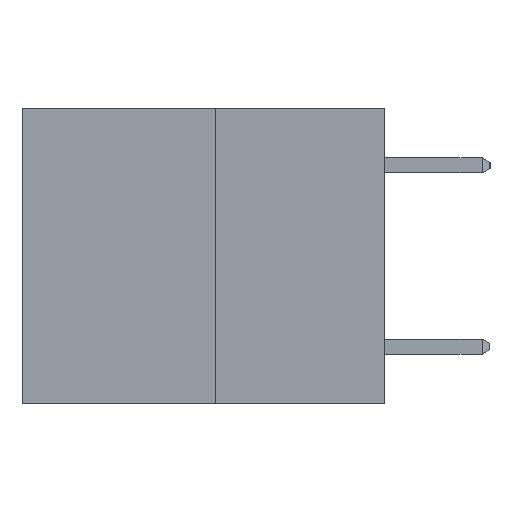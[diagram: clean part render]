
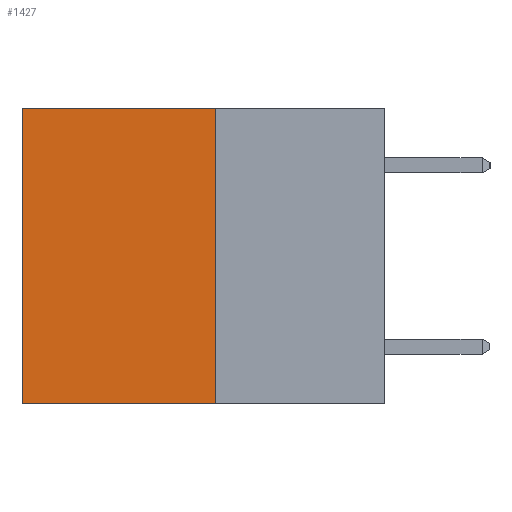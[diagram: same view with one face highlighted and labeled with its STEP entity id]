
A CAD part, left-side view. The second image highlights one B-rep face of the part: STEP entity #1427.
In plain terms, the highlighted planar face has unit normal (-1, 0, 0).
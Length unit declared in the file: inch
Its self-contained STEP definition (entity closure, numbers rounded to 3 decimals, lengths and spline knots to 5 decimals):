
#257 = CARTESIAN_POINT ( 'NONE',  ( 0.3165, 0.6, -0.49 ) ) ;
#453 = CARTESIAN_POINT ( 'NONE',  ( 0.3165, 0.28, 0. ) ) ;
#1127 = PLANE ( 'NONE',  #2078 ) ;
#1200 = LINE ( 'NONE', #2493, #6052 ) ;
#1427 = ADVANCED_FACE ( 'NONE', ( #3220 ), #1127, .F. ) ;
#1482 = EDGE_CURVE ( 'NONE', #6017, #5629, #5645, .T. ) ;
#1552 = ORIENTED_EDGE ( 'NONE', *, *, #5616, .T. ) ;
#2078 = AXIS2_PLACEMENT_3D ( 'NONE', #8502, #3568, #4407 ) ;
#2493 = CARTESIAN_POINT ( 'NONE',  ( 0.3165, 0.28, -0.49 ) ) ;
#3220 = FACE_OUTER_BOUND ( 'NONE', #8354, .T. ) ;
#3568 = DIRECTION ( 'NONE',  ( 1., 0., 0. ) ) ;
#4062 = DIRECTION ( 'NONE',  ( 0., 0., -1. ) ) ;
#4073 = CARTESIAN_POINT ( 'NONE',  ( 0.3165, 0.28, -0.49 ) ) ;
#4407 = DIRECTION ( 'NONE',  ( 0., 0., -1. ) ) ;
#4700 = CARTESIAN_POINT ( 'NONE',  ( 0.3165, 0.6, -0.49 ) ) ;
#4723 = VERTEX_POINT ( 'NONE', #453 ) ;
#4753 = LINE ( 'NONE', #8108, #9536 ) ;
#5454 = LINE ( 'NONE', #4073, #7257 ) ;
#5616 = EDGE_CURVE ( 'NONE', #4723, #6017, #4753, .T. ) ;
#5629 = VERTEX_POINT ( 'NONE', #257 ) ;
#5645 = LINE ( 'NONE', #4700, #7568 ) ;
#5780 = EDGE_CURVE ( 'NONE', #4723, #6565, #1200, .T. ) ;
#6017 = VERTEX_POINT ( 'NONE', #7781 ) ;
#6052 = VECTOR ( 'NONE', #4062, 39.37008 ) ;
#6565 = VERTEX_POINT ( 'NONE', #8383 ) ;
#6800 = EDGE_CURVE ( 'NONE', #6565, #5629, #5454, .T. ) ;
#7257 = VECTOR ( 'NONE', #8183, 39.37008 ) ;
#7568 = VECTOR ( 'NONE', #10477, 39.37008 ) ;
#7781 = CARTESIAN_POINT ( 'NONE',  ( 0.3165, 0.6, 0. ) ) ;
#8108 = CARTESIAN_POINT ( 'NONE',  ( 0.3165, 0.28, 0. ) ) ;
#8158 = DIRECTION ( 'NONE',  ( 0., 1., 0. ) ) ;
#8183 = DIRECTION ( 'NONE',  ( 0., 1., 0. ) ) ;
#8354 = EDGE_LOOP ( 'NONE', ( #9831, #10308, #9812, #1552 ) ) ;
#8383 = CARTESIAN_POINT ( 'NONE',  ( 0.3165, 0.28, -0.49 ) ) ;
#8502 = CARTESIAN_POINT ( 'NONE',  ( 0.3165, 0.28, -0.49 ) ) ;
#9536 = VECTOR ( 'NONE', #8158, 39.37008 ) ;
#9812 = ORIENTED_EDGE ( 'NONE', *, *, #5780, .F. ) ;
#9831 = ORIENTED_EDGE ( 'NONE', *, *, #1482, .T. ) ;
#10308 = ORIENTED_EDGE ( 'NONE', *, *, #6800, .F. ) ;
#10477 = DIRECTION ( 'NONE',  ( 0., 0., -1. ) ) ;
